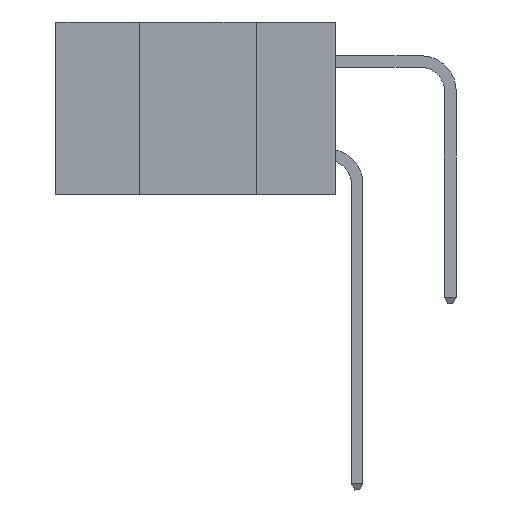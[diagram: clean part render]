
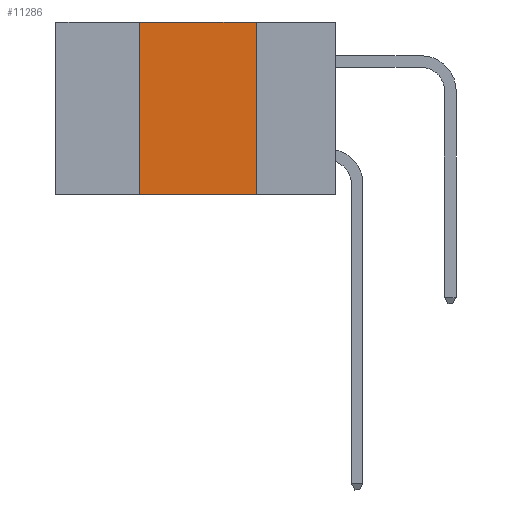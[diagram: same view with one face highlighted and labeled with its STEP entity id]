
A CAD part, left-side view. The second image highlights one B-rep face of the part: STEP entity #11286.
In plain terms, the highlighted planar face has unit normal (-1, 0, 0).
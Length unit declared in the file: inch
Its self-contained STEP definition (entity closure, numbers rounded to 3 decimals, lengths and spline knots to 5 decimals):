
#752 = EDGE_CURVE ( 'NONE', #2003, #3732, #23909, .T. ) ;
#845 = LINE ( 'NONE', #16800, #23891 ) ;
#1182 = CARTESIAN_POINT ( 'NONE',  ( 0., 0.17, 0. ) ) ;
#1208 = EDGE_CURVE ( 'NONE', #2003, #20360, #845, .T. ) ;
#1489 = PLANE ( 'NONE',  #8948 ) ;
#2003 = VERTEX_POINT ( 'NONE', #3002 ) ;
#2306 = LINE ( 'NONE', #1182, #16797 ) ;
#2595 = ORIENTED_EDGE ( 'NONE', *, *, #21296, .F. ) ;
#3002 = CARTESIAN_POINT ( 'NONE',  ( 0., 0.42, -0.37 ) ) ;
#3127 = DIRECTION ( 'NONE',  ( 0., 0., 1. ) ) ;
#3732 = VERTEX_POINT ( 'NONE', #9959 ) ;
#5230 = CARTESIAN_POINT ( 'NONE',  ( 0., 0.17, 0. ) ) ;
#5929 = DIRECTION ( 'NONE',  ( 0., -1., 0. ) ) ;
#6804 = ORIENTED_EDGE ( 'NONE', *, *, #1208, .F. ) ;
#6928 = FACE_OUTER_BOUND ( 'NONE', #10818, .T. ) ;
#7318 = CARTESIAN_POINT ( 'NONE',  ( 0., 0.6, 0. ) ) ;
#7727 = CARTESIAN_POINT ( 'NONE',  ( 0., 0.42, 0. ) ) ;
#8913 = DIRECTION ( 'NONE',  ( 0., 0., -1. ) ) ;
#8948 = AXIS2_PLACEMENT_3D ( 'NONE', #18476, #23892, #13033 ) ;
#9206 = DIRECTION ( 'NONE',  ( 0., -1., 0. ) ) ;
#9959 = CARTESIAN_POINT ( 'NONE',  ( 0., 0.17, -0.37 ) ) ;
#10633 = ORIENTED_EDGE ( 'NONE', *, *, #752, .T. ) ;
#10818 = EDGE_LOOP ( 'NONE', ( #2595, #12433, #6804, #10633 ) ) ;
#11286 = ADVANCED_FACE ( 'NONE', ( #6928 ), #1489, .F. ) ;
#12064 = VERTEX_POINT ( 'NONE', #5230 ) ;
#12433 = ORIENTED_EDGE ( 'NONE', *, *, #22041, .F. ) ;
#13033 = DIRECTION ( 'NONE',  ( 0., 0., -1. ) ) ;
#13091 = CARTESIAN_POINT ( 'NONE',  ( 0., 0.6, -0.37 ) ) ;
#13600 = VECTOR ( 'NONE', #9206, 39.37008 ) ;
#16797 = VECTOR ( 'NONE', #8913, 39.37008 ) ;
#16800 = CARTESIAN_POINT ( 'NONE',  ( 0., 0.42, 0. ) ) ;
#18476 = CARTESIAN_POINT ( 'NONE',  ( 0., 0.6, 0. ) ) ;
#19117 = VECTOR ( 'NONE', #5929, 39.37008 ) ;
#20360 = VERTEX_POINT ( 'NONE', #7727 ) ;
#21296 = EDGE_CURVE ( 'NONE', #12064, #3732, #2306, .T. ) ;
#22041 = EDGE_CURVE ( 'NONE', #20360, #12064, #23789, .T. ) ;
#23789 = LINE ( 'NONE', #7318, #13600 ) ;
#23891 = VECTOR ( 'NONE', #3127, 39.37008 ) ;
#23892 = DIRECTION ( 'NONE',  ( 1., 0., 0. ) ) ;
#23909 = LINE ( 'NONE', #13091, #19117 ) ;
